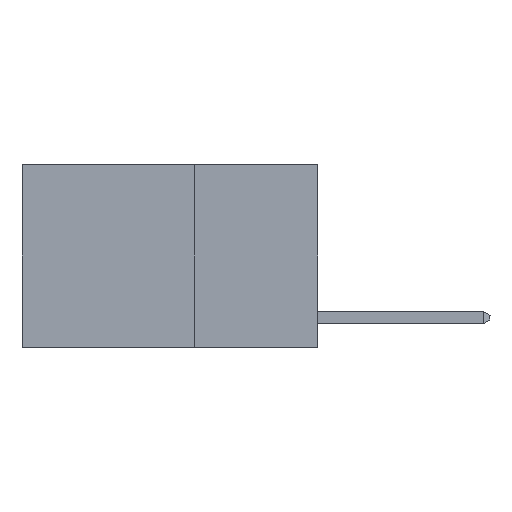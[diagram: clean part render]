
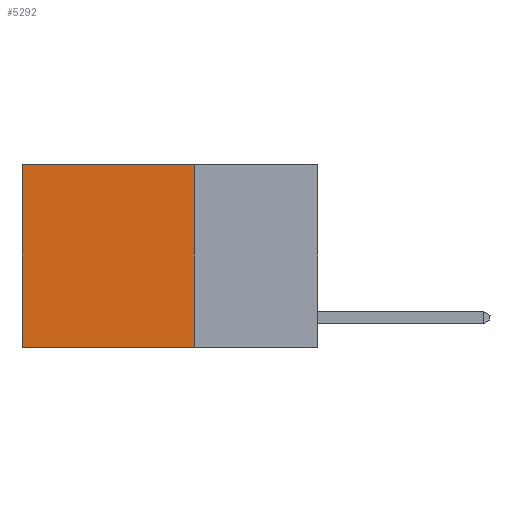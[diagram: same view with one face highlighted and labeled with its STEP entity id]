
A CAD part, left-side view. The second image highlights one B-rep face of the part: STEP entity #5292.
In plain terms, the highlighted planar face has unit normal (-1, 0, 0).
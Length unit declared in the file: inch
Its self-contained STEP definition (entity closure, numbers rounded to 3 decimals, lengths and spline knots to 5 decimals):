
#66 = DIRECTION ( 'NONE',  ( 0., 0., -1. ) ) ;
#395 = CARTESIAN_POINT ( 'NONE',  ( 0.2625, 0.6, 0. ) ) ;
#642 = AXIS2_PLACEMENT_3D ( 'NONE', #3668, #2208, #5154 ) ;
#698 = ORIENTED_EDGE ( 'NONE', *, *, #7541, .T. ) ;
#1055 = EDGE_CURVE ( 'NONE', #5442, #4132, #7069, .T. ) ;
#1285 = EDGE_LOOP ( 'NONE', ( #698, #5332, #2999, #4805 ) ) ;
#1747 = CARTESIAN_POINT ( 'NONE',  ( 0.2625, 0.25, -0.37 ) ) ;
#2085 = VECTOR ( 'NONE', #6228, 39.37008 ) ;
#2208 = DIRECTION ( 'NONE',  ( 1., 0., 0. ) ) ;
#2893 = VECTOR ( 'NONE', #4264, 39.37008 ) ;
#2999 = ORIENTED_EDGE ( 'NONE', *, *, #1055, .F. ) ;
#3668 = CARTESIAN_POINT ( 'NONE',  ( 0.2625, 0.25, 0. ) ) ;
#3867 = FACE_OUTER_BOUND ( 'NONE', #1285, .T. ) ;
#3933 = LINE ( 'NONE', #7770, #8496 ) ;
#4049 = CARTESIAN_POINT ( 'NONE',  ( 0.2625, 0.25, 0. ) ) ;
#4132 = VERTEX_POINT ( 'NONE', #5848 ) ;
#4203 = CARTESIAN_POINT ( 'NONE',  ( 0.2625, 0.6, -0.37 ) ) ;
#4264 = DIRECTION ( 'NONE',  ( 0., 1., 0. ) ) ;
#4486 = CARTESIAN_POINT ( 'NONE',  ( 0.2625, 0.25, 0. ) ) ;
#4560 = PLANE ( 'NONE',  #642 ) ;
#4562 = VERTEX_POINT ( 'NONE', #395 ) ;
#4805 = ORIENTED_EDGE ( 'NONE', *, *, #7917, .T. ) ;
#5154 = DIRECTION ( 'NONE',  ( 0., 0., -1. ) ) ;
#5230 = VERTEX_POINT ( 'NONE', #4203 ) ;
#5292 = ADVANCED_FACE ( 'NONE', ( #3867 ), #4560, .F. ) ;
#5332 = ORIENTED_EDGE ( 'NONE', *, *, #9250, .F. ) ;
#5442 = VERTEX_POINT ( 'NONE', #4049 ) ;
#5848 = CARTESIAN_POINT ( 'NONE',  ( 0.2625, 0.25, -0.37 ) ) ;
#6159 = VECTOR ( 'NONE', #66, 39.37008 ) ;
#6228 = DIRECTION ( 'NONE',  ( 0., 1., 0. ) ) ;
#6301 = CARTESIAN_POINT ( 'NONE',  ( 0.2625, 0.25, 0. ) ) ;
#7069 = LINE ( 'NONE', #6301, #6159 ) ;
#7341 = DIRECTION ( 'NONE',  ( 0., 0., -1. ) ) ;
#7541 = EDGE_CURVE ( 'NONE', #4562, #5230, #3933, .T. ) ;
#7770 = CARTESIAN_POINT ( 'NONE',  ( 0.2625, 0.6, 0. ) ) ;
#7917 = EDGE_CURVE ( 'NONE', #5442, #4562, #9835, .T. ) ;
#8496 = VECTOR ( 'NONE', #7341, 39.37008 ) ;
#8537 = LINE ( 'NONE', #1747, #2893 ) ;
#9250 = EDGE_CURVE ( 'NONE', #4132, #5230, #8537, .T. ) ;
#9835 = LINE ( 'NONE', #4486, #2085 ) ;
